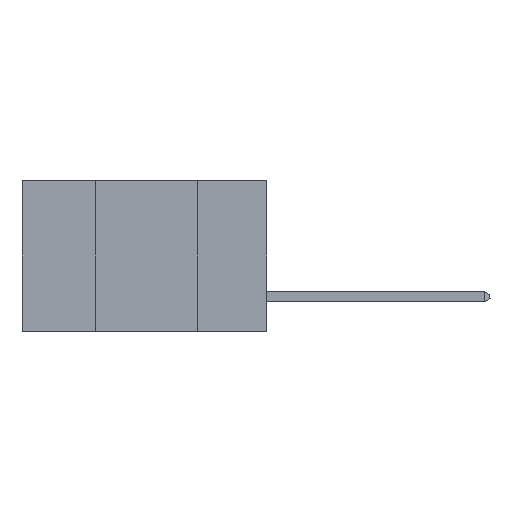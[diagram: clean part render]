
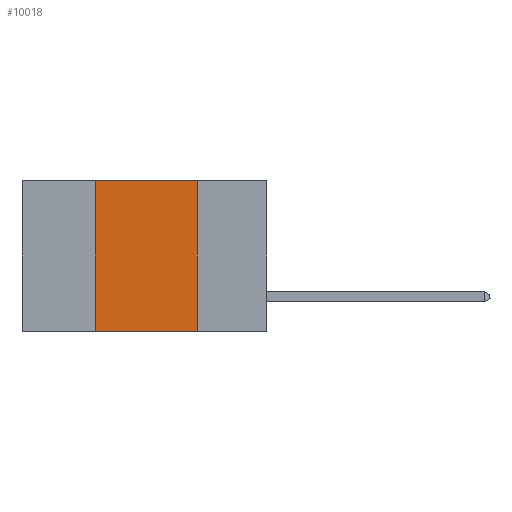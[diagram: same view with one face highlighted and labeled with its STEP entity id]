
A CAD part, left-side view. The second image highlights one B-rep face of the part: STEP entity #10018.
In plain terms, the highlighted planar face has unit normal (-1, 0, 0).
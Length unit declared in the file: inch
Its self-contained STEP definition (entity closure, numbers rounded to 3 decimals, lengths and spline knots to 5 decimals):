
#15 = DIRECTION ( 'NONE',  ( 1., 0., 0. ) ) ;
#310 = EDGE_CURVE ( 'NONE', #4980, #952, #1160, .T. ) ;
#340 = EDGE_LOOP ( 'NONE', ( #8215, #2163, #5023, #2923 ) ) ;
#768 = CARTESIAN_POINT ( 'NONE',  ( 0., 0.42, -0.37 ) ) ;
#952 = VERTEX_POINT ( 'NONE', #7529 ) ;
#1160 = LINE ( 'NONE', #1497, #5297 ) ;
#1497 = CARTESIAN_POINT ( 'NONE',  ( 0., 0.17, 0. ) ) ;
#1622 = PLANE ( 'NONE',  #9622 ) ;
#2163 = ORIENTED_EDGE ( 'NONE', *, *, #5585, .F. ) ;
#2541 = VECTOR ( 'NONE', #3444, 39.37008 ) ;
#2923 = ORIENTED_EDGE ( 'NONE', *, *, #9222, .T. ) ;
#3164 = FACE_OUTER_BOUND ( 'NONE', #340, .T. ) ;
#3444 = DIRECTION ( 'NONE',  ( 0., -1., 0. ) ) ;
#3767 = CARTESIAN_POINT ( 'NONE',  ( 0., 0.17, 0. ) ) ;
#3792 = EDGE_CURVE ( 'NONE', #8060, #6682, #4776, .T. ) ;
#4776 = LINE ( 'NONE', #9668, #6352 ) ;
#4980 = VERTEX_POINT ( 'NONE', #3767 ) ;
#5023 = ORIENTED_EDGE ( 'NONE', *, *, #3792, .F. ) ;
#5297 = VECTOR ( 'NONE', #6955, 39.37008 ) ;
#5585 = EDGE_CURVE ( 'NONE', #6682, #4980, #8882, .T. ) ;
#6352 = VECTOR ( 'NONE', #6568, 39.37008 ) ;
#6568 = DIRECTION ( 'NONE',  ( 0., 0., 1. ) ) ;
#6589 = CARTESIAN_POINT ( 'NONE',  ( 0., 0.6, 0. ) ) ;
#6682 = VERTEX_POINT ( 'NONE', #7555 ) ;
#6955 = DIRECTION ( 'NONE',  ( 0., 0., -1. ) ) ;
#7068 = DIRECTION ( 'NONE',  ( 0., 0., -1. ) ) ;
#7529 = CARTESIAN_POINT ( 'NONE',  ( 0., 0.17, -0.37 ) ) ;
#7555 = CARTESIAN_POINT ( 'NONE',  ( 0., 0.42, 0. ) ) ;
#7763 = VECTOR ( 'NONE', #8879, 39.37008 ) ;
#8060 = VERTEX_POINT ( 'NONE', #768 ) ;
#8147 = LINE ( 'NONE', #8752, #7763 ) ;
#8215 = ORIENTED_EDGE ( 'NONE', *, *, #310, .F. ) ;
#8752 = CARTESIAN_POINT ( 'NONE',  ( 0., 0.6, -0.37 ) ) ;
#8879 = DIRECTION ( 'NONE',  ( 0., -1., 0. ) ) ;
#8882 = LINE ( 'NONE', #6589, #2541 ) ;
#9222 = EDGE_CURVE ( 'NONE', #8060, #952, #8147, .T. ) ;
#9389 = CARTESIAN_POINT ( 'NONE',  ( 0., 0.6, 0. ) ) ;
#9622 = AXIS2_PLACEMENT_3D ( 'NONE', #9389, #15, #7068 ) ;
#9668 = CARTESIAN_POINT ( 'NONE',  ( 0., 0.42, 0. ) ) ;
#10018 = ADVANCED_FACE ( 'NONE', ( #3164 ), #1622, .F. ) ;
